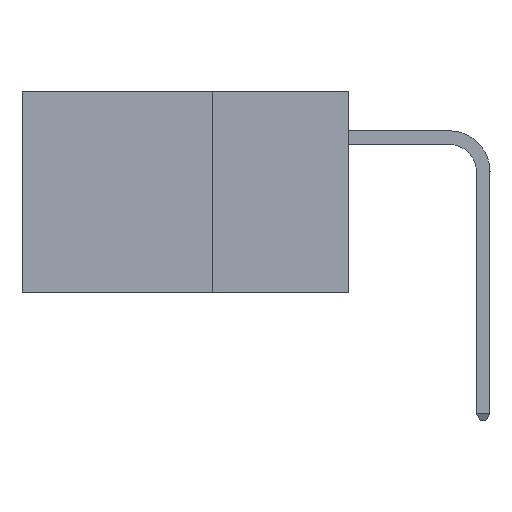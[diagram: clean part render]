
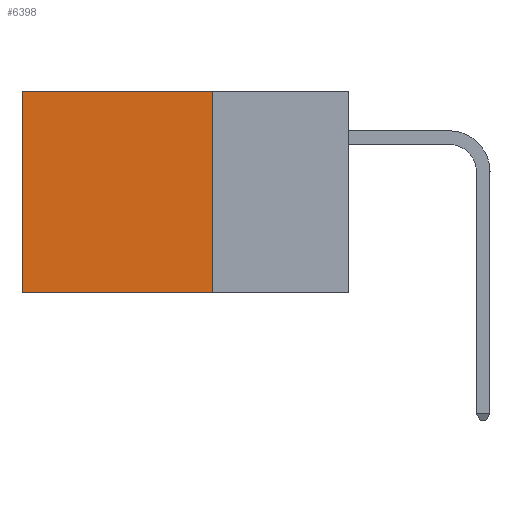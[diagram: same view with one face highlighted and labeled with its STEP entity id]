
A CAD part, left-side view. The second image highlights one B-rep face of the part: STEP entity #6398.
In plain terms, the highlighted planar face has unit normal (-1, 0, 0).
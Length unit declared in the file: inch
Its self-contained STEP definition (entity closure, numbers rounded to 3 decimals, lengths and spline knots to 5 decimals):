
#2141 = EDGE_CURVE ( 'NONE', #2468, #27213, #40446, .T. ) ;
#2468 = VERTEX_POINT ( 'NONE', #13264 ) ;
#2820 = ORIENTED_EDGE ( 'NONE', *, *, #2141, .F. ) ;
#4708 = EDGE_CURVE ( 'NONE', #21836, #27949, #34481, .T. ) ;
#5582 = CARTESIAN_POINT ( 'NONE',  ( 0.2875, 0.25, 0. ) ) ;
#6398 = ADVANCED_FACE ( 'NONE', ( #17063 ), #18893, .F. ) ;
#7304 = DIRECTION ( 'NONE',  ( 0., 1., 0. ) ) ;
#8983 = DIRECTION ( 'NONE',  ( 0., 0., -1. ) ) ;
#13260 = CARTESIAN_POINT ( 'NONE',  ( 0.2875, 0.25, 0. ) ) ;
#13264 = CARTESIAN_POINT ( 'NONE',  ( 0.2875, 0.25, 0. ) ) ;
#14666 = CARTESIAN_POINT ( 'NONE',  ( 0.2875, 0.25, -0.37 ) ) ;
#15486 = VECTOR ( 'NONE', #16580, 39.37008 ) ;
#16249 = ORIENTED_EDGE ( 'NONE', *, *, #4708, .T. ) ;
#16524 = LINE ( 'NONE', #13260, #15486 ) ;
#16550 = CARTESIAN_POINT ( 'NONE',  ( 0.2875, 0.25, 0. ) ) ;
#16580 = DIRECTION ( 'NONE',  ( 0., 1., 0. ) ) ;
#17063 = FACE_OUTER_BOUND ( 'NONE', #18627, .T. ) ;
#18627 = EDGE_LOOP ( 'NONE', ( #16249, #27053, #2820, #22993 ) ) ;
#18711 = EDGE_CURVE ( 'NONE', #2468, #21836, #16524, .T. ) ;
#18893 = PLANE ( 'NONE',  #26341 ) ;
#19627 = CARTESIAN_POINT ( 'NONE',  ( 0.2875, 0.6, 0. ) ) ;
#21836 = VERTEX_POINT ( 'NONE', #19627 ) ;
#22993 = ORIENTED_EDGE ( 'NONE', *, *, #18711, .T. ) ;
#24326 = CARTESIAN_POINT ( 'NONE',  ( 0.2875, 0.6, 0. ) ) ;
#25739 = VECTOR ( 'NONE', #7304, 39.37008 ) ;
#26341 = AXIS2_PLACEMENT_3D ( 'NONE', #5582, #29046, #8983 ) ;
#26802 = LINE ( 'NONE', #34084, #25739 ) ;
#27053 = ORIENTED_EDGE ( 'NONE', *, *, #36692, .F. ) ;
#27213 = VERTEX_POINT ( 'NONE', #14666 ) ;
#27651 = DIRECTION ( 'NONE',  ( 0., 0., -1. ) ) ;
#27949 = VERTEX_POINT ( 'NONE', #28203 ) ;
#28203 = CARTESIAN_POINT ( 'NONE',  ( 0.2875, 0.6, -0.37 ) ) ;
#29046 = DIRECTION ( 'NONE',  ( 1., 0., 0. ) ) ;
#31581 = VECTOR ( 'NONE', #36727, 39.37008 ) ;
#33424 = VECTOR ( 'NONE', #27651, 39.37008 ) ;
#34084 = CARTESIAN_POINT ( 'NONE',  ( 0.2875, 0.25, -0.37 ) ) ;
#34481 = LINE ( 'NONE', #24326, #33424 ) ;
#36692 = EDGE_CURVE ( 'NONE', #27213, #27949, #26802, .T. ) ;
#36727 = DIRECTION ( 'NONE',  ( 0., 0., -1. ) ) ;
#40446 = LINE ( 'NONE', #16550, #31581 ) ;
